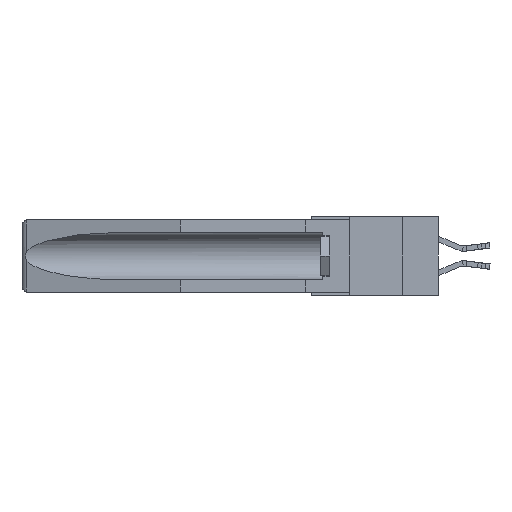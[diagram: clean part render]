
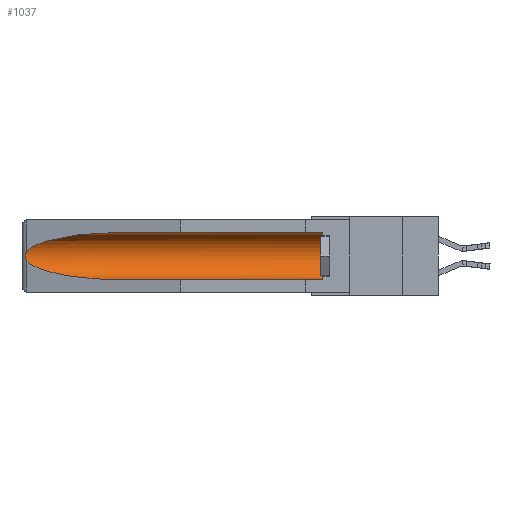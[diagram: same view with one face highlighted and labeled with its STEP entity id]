
A CAD part, left-side view. The second image highlights one B-rep face of the part: STEP entity #1037.
In plain terms, the highlighted cylindrical face has radius 2.857 mm (diameter 5.715 mm), a partial arc.
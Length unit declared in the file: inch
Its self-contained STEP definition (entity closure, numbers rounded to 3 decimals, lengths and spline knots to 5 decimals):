
#296 = EDGE_CURVE ( 'NONE', #20426, #20671, #9444, .T. ) ;
#371 = CARTESIAN_POINT ( 'NONE',  ( 0.26537, 1.52718, -0.14972 ) ) ;
#626 = DIRECTION ( 'NONE',  ( 0., -1., 0. ) ) ;
#670 = AXIS2_PLACEMENT_3D ( 'NONE', #8321, #10750, #1276 ) ;
#777 = CYLINDRICAL_SURFACE ( 'NONE', #670, 0.1125 ) ;
#1037 = ADVANCED_FACE ( 'NONE', ( #24003 ), #777, .F. ) ;
#1044 = CARTESIAN_POINT ( 'NONE',  ( 0.155, 0.126, -0.284 ) ) ;
#1199 = ORIENTED_EDGE ( 'NONE', *, *, #22224, .T. ) ;
#1276 = DIRECTION ( 'NONE',  ( 0., 0., 1. ) ) ;
#1326 =( BOUNDED_CURVE ( )  B_SPLINE_CURVE ( 3, ( #15618, #15716, #10998, #27688 ),
 .UNSPECIFIED., .F., .F. ) 
 B_SPLINE_CURVE_WITH_KNOTS ( ( 4, 4 ),
 ( 0.1948, 1.5708 ),
 .UNSPECIFIED. ) 
 CURVE ( )  GEOMETRIC_REPRESENTATION_ITEM ( )  RATIONAL_B_SPLINE_CURVE ( ( 1., 0.848, 0.848, 1. ) ) 
 REPRESENTATION_ITEM ( '' )  );
#1475 = VERTEX_POINT ( 'NONE', #22714 ) ;
#2562 = CARTESIAN_POINT ( 'NONE',  ( 0.26537, 1.52718, -0.14972 ) ) ;
#2911 = DIRECTION ( 'NONE',  ( 0., 1., 0. ) ) ;
#4592 = CARTESIAN_POINT ( 'NONE',  ( 0.26537, 1.52718, -0.19328 ) ) ;
#4946 = VERTEX_POINT ( 'NONE', #1044 ) ;
#5096 = DIRECTION ( 'NONE',  ( 0., 0., 1. ) ) ;
#7599 = CARTESIAN_POINT ( 'NONE',  ( 0.2675, 1.53308, -0.17534 ) ) ;
#7747 = DIRECTION ( 'NONE',  ( 0., 1., 0. ) ) ;
#7809 = CARTESIAN_POINT ( 'NONE',  ( 0.26654, 1.53092, -0.15636 ) ) ;
#8321 = CARTESIAN_POINT ( 'NONE',  ( 0.155, -0.30754, -0.1715 ) ) ;
#9444 = B_SPLINE_CURVE_WITH_KNOTS ( 'NONE', 3,
 ( #371, #22146, #7809, #17048, #10259, #7599, #10040, #26728, #26829, #12469 ),
 .UNSPECIFIED., .F., .F.,
 ( 4, 2, 2, 2, 4 ),
 ( 0., 0.00029, 0.00058, 0.00087, 0.00117 ),
 .UNSPECIFIED. ) ;
#10040 = CARTESIAN_POINT ( 'NONE',  ( 0.2673, 1.53269, -0.17917 ) ) ;
#10189 =( BOUNDED_CURVE ( )  B_SPLINE_CURVE ( 3, ( #11062, #13279, #11268, #13476 ),
 .UNSPECIFIED., .F., .T. ) 
 B_SPLINE_CURVE_WITH_KNOTS ( ( 4, 4 ),
 ( 4.71239, 6.08839 ),
 .UNSPECIFIED. ) 
 CURVE ( )  GEOMETRIC_REPRESENTATION_ITEM ( )  RATIONAL_B_SPLINE_CURVE ( ( 1., 0.848, 0.848, 1. ) ) 
 REPRESENTATION_ITEM ( '' )  );
#10239 = ORIENTED_EDGE ( 'NONE', *, *, #12322, .F. ) ;
#10259 = CARTESIAN_POINT ( 'NONE',  ( 0.2675, 1.53308, -0.16763 ) ) ;
#10520 = CARTESIAN_POINT ( 'NONE',  ( 0.155, -0.30754, -0.284 ) ) ;
#10750 = DIRECTION ( 'NONE',  ( 0., 1., 0. ) ) ;
#10998 = CARTESIAN_POINT ( 'NONE',  ( 0.21114, 1.30732, -0.284 ) ) ;
#11062 = CARTESIAN_POINT ( 'NONE',  ( 0.155, 1.07973, -0.059 ) ) ;
#11268 = CARTESIAN_POINT ( 'NONE',  ( 0.25451, 1.48313, -0.09465 ) ) ;
#11412 = EDGE_CURVE ( 'NONE', #4946, #1475, #20747, .T. ) ;
#11870 = ORIENTED_EDGE ( 'NONE', *, *, #296, .T. ) ;
#12322 = EDGE_CURVE ( 'NONE', #4946, #15884, #28141, .T. ) ;
#12469 = CARTESIAN_POINT ( 'NONE',  ( 0.26537, 1.52718, -0.19328 ) ) ;
#12748 = VECTOR ( 'NONE', #2911, 39.37008 ) ;
#13279 = CARTESIAN_POINT ( 'NONE',  ( 0.21114, 1.30732, -0.059 ) ) ;
#13319 = EDGE_LOOP ( 'NONE', ( #1199, #11870, #16431, #10239, #26825, #16217 ) ) ;
#13476 = CARTESIAN_POINT ( 'NONE',  ( 0.26537, 1.52718, -0.14972 ) ) ;
#14364 = VECTOR ( 'NONE', #7747, 39.37008 ) ;
#14621 = EDGE_CURVE ( 'NONE', #1475, #23458, #29510, .T. ) ;
#15618 = CARTESIAN_POINT ( 'NONE',  ( 0.26537, 1.52718, -0.19328 ) ) ;
#15716 = CARTESIAN_POINT ( 'NONE',  ( 0.25451, 1.48313, -0.24835 ) ) ;
#15884 = VERTEX_POINT ( 'NONE', #28572 ) ;
#16217 = ORIENTED_EDGE ( 'NONE', *, *, #14621, .T. ) ;
#16431 = ORIENTED_EDGE ( 'NONE', *, *, #16882, .T. ) ;
#16882 = EDGE_CURVE ( 'NONE', #20671, #15884, #1326, .T. ) ;
#17048 = CARTESIAN_POINT ( 'NONE',  ( 0.2673, 1.5327, -0.16383 ) ) ;
#17984 = CARTESIAN_POINT ( 'NONE',  ( 0.155, 1.07973, -0.059 ) ) ;
#20426 = VERTEX_POINT ( 'NONE', #2562 ) ;
#20671 = VERTEX_POINT ( 'NONE', #4592 ) ;
#20747 = CIRCLE ( 'NONE', #26692, 0.1125 ) ;
#22146 = CARTESIAN_POINT ( 'NONE',  ( 0.26597, 1.52961, -0.15275 ) ) ;
#22224 = EDGE_CURVE ( 'NONE', #23458, #20426, #10189, .T. ) ;
#22302 = CARTESIAN_POINT ( 'NONE',  ( 0.155, 0.126, -0.1715 ) ) ;
#22714 = CARTESIAN_POINT ( 'NONE',  ( 0.155, 0.126, -0.059 ) ) ;
#23458 = VERTEX_POINT ( 'NONE', #17984 ) ;
#24003 = FACE_OUTER_BOUND ( 'NONE', #13319, .T. ) ;
#24478 = CARTESIAN_POINT ( 'NONE',  ( 0.155, -0.30754, -0.059 ) ) ;
#26692 = AXIS2_PLACEMENT_3D ( 'NONE', #22302, #626, #5096 ) ;
#26728 = CARTESIAN_POINT ( 'NONE',  ( 0.26655, 1.53094, -0.18657 ) ) ;
#26825 = ORIENTED_EDGE ( 'NONE', *, *, #11412, .T. ) ;
#26829 = CARTESIAN_POINT ( 'NONE',  ( 0.26597, 1.5296, -0.19026 ) ) ;
#27688 = CARTESIAN_POINT ( 'NONE',  ( 0.155, 1.07973, -0.284 ) ) ;
#28141 = LINE ( 'NONE', #10520, #14364 ) ;
#28572 = CARTESIAN_POINT ( 'NONE',  ( 0.155, 1.07973, -0.284 ) ) ;
#29510 = LINE ( 'NONE', #24478, #12748 ) ;
